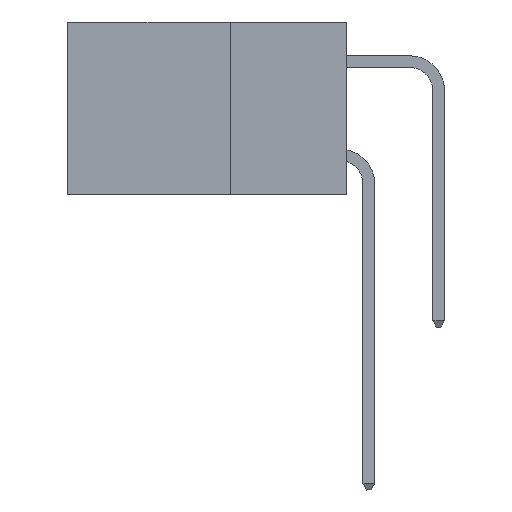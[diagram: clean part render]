
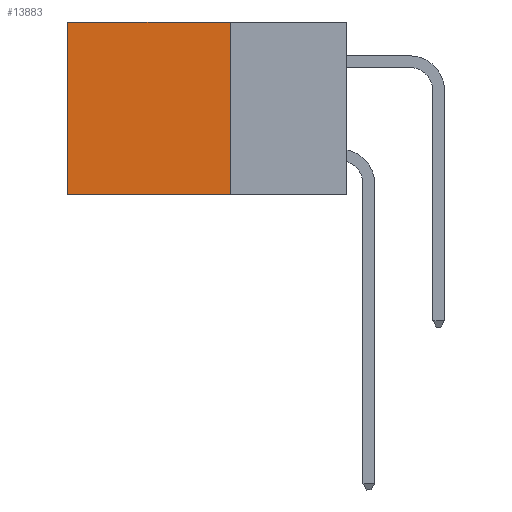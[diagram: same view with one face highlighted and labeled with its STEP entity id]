
A CAD part, left-side view. The second image highlights one B-rep face of the part: STEP entity #13883.
In plain terms, the highlighted planar face has unit normal (-1, 0, 0).
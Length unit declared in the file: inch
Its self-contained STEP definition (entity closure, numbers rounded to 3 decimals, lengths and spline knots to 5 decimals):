
#109 = AXIS2_PLACEMENT_3D ( 'NONE', #8865, #13334, #4269 ) ;
#285 = CARTESIAN_POINT ( 'NONE',  ( 0.2875, 0.25, 0. ) ) ;
#791 = EDGE_CURVE ( 'NONE', #12020, #17075, #18089, .T. ) ;
#976 = EDGE_CURVE ( 'NONE', #12958, #9895, #3287, .T. ) ;
#1335 = CARTESIAN_POINT ( 'NONE',  ( 0.2875, 0.25, -0.37 ) ) ;
#1896 = DIRECTION ( 'NONE',  ( 0., 0., -1. ) ) ;
#2674 = PLANE ( 'NONE',  #109 ) ;
#2918 = DIRECTION ( 'NONE',  ( 0., 1., 0. ) ) ;
#3287 = LINE ( 'NONE', #285, #10550 ) ;
#3597 = CARTESIAN_POINT ( 'NONE',  ( 0.2875, 0.25, 0. ) ) ;
#4269 = DIRECTION ( 'NONE',  ( 0., 0., -1. ) ) ;
#4479 = CARTESIAN_POINT ( 'NONE',  ( 0.2875, 0.6, -0.37 ) ) ;
#4642 = DIRECTION ( 'NONE',  ( 0., 1., 0. ) ) ;
#5579 = EDGE_CURVE ( 'NONE', #9895, #17075, #10399, .T. ) ;
#6231 = VECTOR ( 'NONE', #12151, 39.37008 ) ;
#8493 = ORIENTED_EDGE ( 'NONE', *, *, #976, .F. ) ;
#8865 = CARTESIAN_POINT ( 'NONE',  ( 0.2875, 0.25, 0. ) ) ;
#9373 = CARTESIAN_POINT ( 'NONE',  ( 0.2875, 0.6, 0. ) ) ;
#9895 = VERTEX_POINT ( 'NONE', #18979 ) ;
#10317 = ORIENTED_EDGE ( 'NONE', *, *, #14741, .T. ) ;
#10399 = LINE ( 'NONE', #1335, #17719 ) ;
#10550 = VECTOR ( 'NONE', #1896, 39.37008 ) ;
#10783 = ORIENTED_EDGE ( 'NONE', *, *, #5579, .F. ) ;
#11964 = LINE ( 'NONE', #18088, #19280 ) ;
#12020 = VERTEX_POINT ( 'NONE', #9373 ) ;
#12074 = EDGE_LOOP ( 'NONE', ( #19213, #10783, #8493, #10317 ) ) ;
#12151 = DIRECTION ( 'NONE',  ( 0., 0., -1. ) ) ;
#12958 = VERTEX_POINT ( 'NONE', #3597 ) ;
#13334 = DIRECTION ( 'NONE',  ( 1., 0., 0. ) ) ;
#13883 = ADVANCED_FACE ( 'NONE', ( #15605 ), #2674, .F. ) ;
#14741 = EDGE_CURVE ( 'NONE', #12958, #12020, #11964, .T. ) ;
#15432 = CARTESIAN_POINT ( 'NONE',  ( 0.2875, 0.6, 0. ) ) ;
#15605 = FACE_OUTER_BOUND ( 'NONE', #12074, .T. ) ;
#17075 = VERTEX_POINT ( 'NONE', #4479 ) ;
#17719 = VECTOR ( 'NONE', #2918, 39.37008 ) ;
#18088 = CARTESIAN_POINT ( 'NONE',  ( 0.2875, 0.25, 0. ) ) ;
#18089 = LINE ( 'NONE', #15432, #6231 ) ;
#18979 = CARTESIAN_POINT ( 'NONE',  ( 0.2875, 0.25, -0.37 ) ) ;
#19213 = ORIENTED_EDGE ( 'NONE', *, *, #791, .T. ) ;
#19280 = VECTOR ( 'NONE', #4642, 39.37008 ) ;
